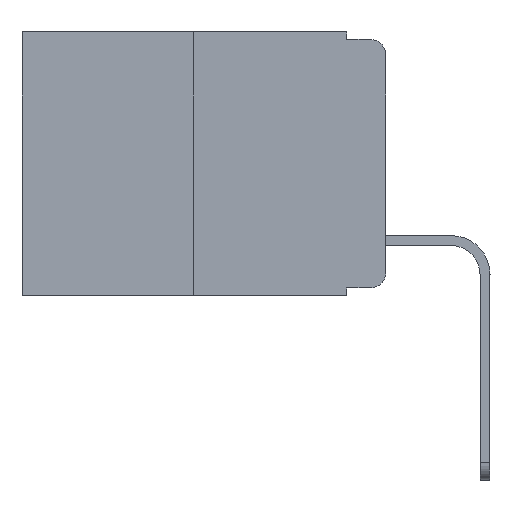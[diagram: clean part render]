
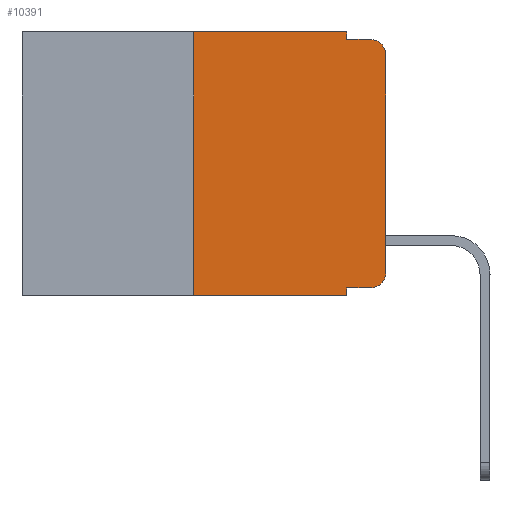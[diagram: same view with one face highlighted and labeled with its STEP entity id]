
A CAD part, left-side view. The second image highlights one B-rep face of the part: STEP entity #10391.
In plain terms, the highlighted planar face has unit normal (-1, 0, 0).
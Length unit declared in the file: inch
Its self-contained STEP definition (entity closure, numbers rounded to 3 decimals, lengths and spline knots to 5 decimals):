
#15 = CARTESIAN_POINT ( 'NONE',  ( 0., 0., -0.313 ) ) ;
#26 = CARTESIAN_POINT ( 'NONE',  ( 0., 0., -0.03 ) ) ;
#148 = CARTESIAN_POINT ( 'NONE',  ( 0., 0.051, -0.343 ) ) ;
#248 = CARTESIAN_POINT ( 'NONE',  ( 0., 0.473, 0. ) ) ;
#343 = VERTEX_POINT ( 'NONE', #9499 ) ;
#484 = DIRECTION ( 'NONE',  ( 0., 0., -1. ) ) ;
#643 = VERTEX_POINT ( 'NONE', #1144 ) ;
#729 = VECTOR ( 'NONE', #8138, 39.37008 ) ;
#1144 = CARTESIAN_POINT ( 'NONE',  ( 0., 0.051, -0.333 ) ) ;
#1287 = VERTEX_POINT ( 'NONE', #6237 ) ;
#1586 = VECTOR ( 'NONE', #10022, 39.37008 ) ;
#1874 = CARTESIAN_POINT ( 'NONE',  ( 0., 0.02, -0.333 ) ) ;
#1988 = CARTESIAN_POINT ( 'NONE',  ( 0., 0.051, 0. ) ) ;
#2233 = CARTESIAN_POINT ( 'NONE',  ( 0., 0.051, -0.01 ) ) ;
#2335 = VECTOR ( 'NONE', #2463, 39.37008 ) ;
#2463 = DIRECTION ( 'NONE',  ( 0., 0., -1. ) ) ;
#2546 = CARTESIAN_POINT ( 'NONE',  ( 0., 0.051, 0. ) ) ;
#2878 = EDGE_CURVE ( 'NONE', #1287, #4710, #11841, .T. ) ;
#3310 = CARTESIAN_POINT ( 'NONE',  ( 0., 0.25, 0. ) ) ;
#3342 = AXIS2_PLACEMENT_3D ( 'NONE', #11048, #7238, #9139 ) ;
#3471 = EDGE_CURVE ( 'NONE', #4072, #6754, #7235, .T. ) ;
#3648 = AXIS2_PLACEMENT_3D ( 'NONE', #4319, #12134, #484 ) ;
#3853 = LINE ( 'NONE', #9455, #4156 ) ;
#3923 = EDGE_CURVE ( 'NONE', #643, #4710, #3853, .T. ) ;
#3966 = DIRECTION ( 'NONE',  ( 0., 0., -1. ) ) ;
#4072 = VERTEX_POINT ( 'NONE', #15 ) ;
#4104 = VECTOR ( 'NONE', #10624, 39.37008 ) ;
#4156 = VECTOR ( 'NONE', #3966, 39.37008 ) ;
#4319 = CARTESIAN_POINT ( 'NONE',  ( 0., 0.02, -0.03 ) ) ;
#4640 = CIRCLE ( 'NONE', #3342, 0.02 ) ;
#4645 = VECTOR ( 'NONE', #9232, 39.37008 ) ;
#4710 = VERTEX_POINT ( 'NONE', #148 ) ;
#5048 = DIRECTION ( 'NONE',  ( 0., -1., 0. ) ) ;
#5449 = VERTEX_POINT ( 'NONE', #1874 ) ;
#5779 = CIRCLE ( 'NONE', #3648, 0.02 ) ;
#6109 = ORIENTED_EDGE ( 'NONE', *, *, #11836, .T. ) ;
#6112 = CARTESIAN_POINT ( 'NONE',  ( 0., 0.051, -0.01 ) ) ;
#6237 = CARTESIAN_POINT ( 'NONE',  ( 0., 0.25, -0.343 ) ) ;
#6352 = EDGE_CURVE ( 'NONE', #8204, #11101, #10476, .T. ) ;
#6754 = VERTEX_POINT ( 'NONE', #26 ) ;
#6756 = DIRECTION ( 'NONE',  ( 0., 0., -1. ) ) ;
#7170 = LINE ( 'NONE', #7898, #11748 ) ;
#7235 = LINE ( 'NONE', #7347, #4645 ) ;
#7238 = DIRECTION ( 'NONE',  ( -1., 0., 0. ) ) ;
#7306 = ORIENTED_EDGE ( 'NONE', *, *, #8037, .T. ) ;
#7347 = CARTESIAN_POINT ( 'NONE',  ( 0., 0., 0. ) ) ;
#7380 = LINE ( 'NONE', #2233, #1586 ) ;
#7584 = ORIENTED_EDGE ( 'NONE', *, *, #3923, .F. ) ;
#7607 = ORIENTED_EDGE ( 'NONE', *, *, #2878, .T. ) ;
#7716 = ORIENTED_EDGE ( 'NONE', *, *, #9792, .T. ) ;
#7898 = CARTESIAN_POINT ( 'NONE',  ( 0., 0.051, -0.333 ) ) ;
#8037 = EDGE_CURVE ( 'NONE', #643, #5449, #7170, .T. ) ;
#8138 = DIRECTION ( 'NONE',  ( 0., -1., 0. ) ) ;
#8148 = VERTEX_POINT ( 'NONE', #6112 ) ;
#8190 = CARTESIAN_POINT ( 'NONE',  ( 0., 0.473, -0.343 ) ) ;
#8204 = VERTEX_POINT ( 'NONE', #3310 ) ;
#8414 = EDGE_CURVE ( 'NONE', #1287, #8204, #12206, .T. ) ;
#8796 = ORIENTED_EDGE ( 'NONE', *, *, #8414, .F. ) ;
#9139 = DIRECTION ( 'NONE',  ( 0., 0., -1. ) ) ;
#9182 = LINE ( 'NONE', #2546, #2335 ) ;
#9198 = VECTOR ( 'NONE', #12084, 39.37008 ) ;
#9232 = DIRECTION ( 'NONE',  ( 0., 0., 1. ) ) ;
#9455 = CARTESIAN_POINT ( 'NONE',  ( 0., 0.051, 0. ) ) ;
#9499 = CARTESIAN_POINT ( 'NONE',  ( 0., 0.02, -0.01 ) ) ;
#9600 = CARTESIAN_POINT ( 'NONE',  ( 0., 0.473, 0. ) ) ;
#9639 = FACE_OUTER_BOUND ( 'NONE', #10818, .T. ) ;
#9792 = EDGE_CURVE ( 'NONE', #6754, #343, #5779, .T. ) ;
#10008 = ORIENTED_EDGE ( 'NONE', *, *, #12280, .F. ) ;
#10021 = ORIENTED_EDGE ( 'NONE', *, *, #11948, .F. ) ;
#10022 = DIRECTION ( 'NONE',  ( 0., -1., 0. ) ) ;
#10172 = ORIENTED_EDGE ( 'NONE', *, *, #6352, .F. ) ;
#10391 = ADVANCED_FACE ( 'NONE', ( #9639 ), #11603, .F. ) ;
#10476 = LINE ( 'NONE', #248, #729 ) ;
#10624 = DIRECTION ( 'NONE',  ( 0., 0., 1. ) ) ;
#10818 = EDGE_LOOP ( 'NONE', ( #11606, #7716, #10008, #10021, #10172, #8796, #7607, #7584, #7306, #6109 ) ) ;
#11048 = CARTESIAN_POINT ( 'NONE',  ( 0., 0.02, -0.313 ) ) ;
#11101 = VERTEX_POINT ( 'NONE', #1988 ) ;
#11401 = AXIS2_PLACEMENT_3D ( 'NONE', #9600, #11553, #6756 ) ;
#11553 = DIRECTION ( 'NONE',  ( 1., 0., 0. ) ) ;
#11603 = PLANE ( 'NONE',  #11401 ) ;
#11606 = ORIENTED_EDGE ( 'NONE', *, *, #3471, .T. ) ;
#11657 = CARTESIAN_POINT ( 'NONE',  ( 0., 0.25, 0. ) ) ;
#11748 = VECTOR ( 'NONE', #5048, 39.37008 ) ;
#11836 = EDGE_CURVE ( 'NONE', #5449, #4072, #4640, .T. ) ;
#11841 = LINE ( 'NONE', #8190, #9198 ) ;
#11948 = EDGE_CURVE ( 'NONE', #11101, #8148, #9182, .T. ) ;
#12084 = DIRECTION ( 'NONE',  ( 0., -1., 0. ) ) ;
#12134 = DIRECTION ( 'NONE',  ( -1., 0., 0. ) ) ;
#12206 = LINE ( 'NONE', #11657, #4104 ) ;
#12280 = EDGE_CURVE ( 'NONE', #8148, #343, #7380, .T. ) ;
